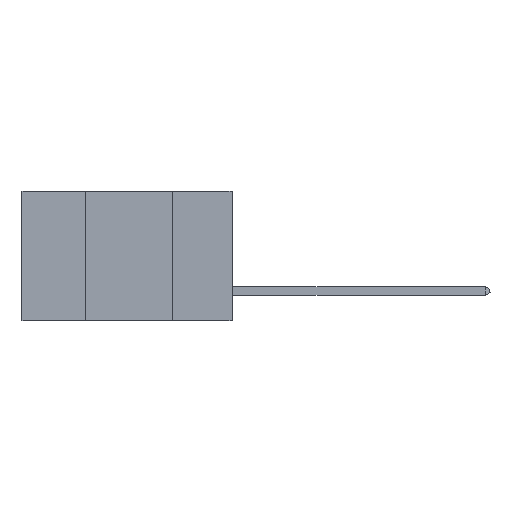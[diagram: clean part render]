
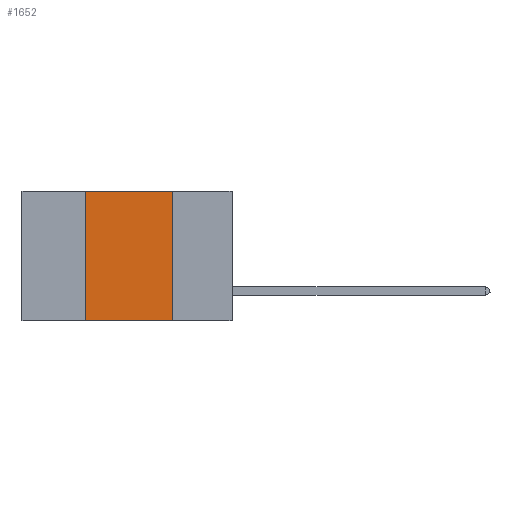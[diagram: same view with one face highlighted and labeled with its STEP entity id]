
A CAD part, left-side view. The second image highlights one B-rep face of the part: STEP entity #1652.
In plain terms, the highlighted planar face has unit normal (-1, 0, 0).
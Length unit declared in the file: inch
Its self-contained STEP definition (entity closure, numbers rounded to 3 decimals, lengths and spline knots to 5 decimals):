
#107 = PLANE ( 'NONE',  #6548 ) ;
#110 = VERTEX_POINT ( 'NONE', #2593 ) ;
#738 = ORIENTED_EDGE ( 'NONE', *, *, #14690, .T. ) ;
#1109 = LINE ( 'NONE', #14094, #13991 ) ;
#1227 = CARTESIAN_POINT ( 'NONE',  ( 0., 0.17, 0. ) ) ;
#1652 = ADVANCED_FACE ( 'NONE', ( #6645 ), #107, .F. ) ;
#2269 = ORIENTED_EDGE ( 'NONE', *, *, #9632, .F. ) ;
#2276 = VERTEX_POINT ( 'NONE', #3447 ) ;
#2307 = EDGE_CURVE ( 'NONE', #13519, #12713, #13987, .T. ) ;
#2593 = CARTESIAN_POINT ( 'NONE',  ( 0., 0.42, -0.37 ) ) ;
#3060 = LINE ( 'NONE', #14406, #4971 ) ;
#3086 = EDGE_CURVE ( 'NONE', #110, #2276, #1109, .T. ) ;
#3099 = EDGE_LOOP ( 'NONE', ( #4401, #2269, #9036, #738 ) ) ;
#3417 = DIRECTION ( 'NONE',  ( 0., -1., 0. ) ) ;
#3447 = CARTESIAN_POINT ( 'NONE',  ( 0., 0.42, 0. ) ) ;
#3971 = DIRECTION ( 'NONE',  ( 1., 0., 0. ) ) ;
#4401 = ORIENTED_EDGE ( 'NONE', *, *, #2307, .F. ) ;
#4971 = VECTOR ( 'NONE', #6022, 39.37008 ) ;
#5076 = CARTESIAN_POINT ( 'NONE',  ( 0., 0.6, 0. ) ) ;
#5434 = CARTESIAN_POINT ( 'NONE',  ( 0., 0.17, -0.37 ) ) ;
#5524 = DIRECTION ( 'NONE',  ( 0., 0., 1. ) ) ;
#6022 = DIRECTION ( 'NONE',  ( 0., -1., 0. ) ) ;
#6548 = AXIS2_PLACEMENT_3D ( 'NONE', #5076, #3971, #14720 ) ;
#6645 = FACE_OUTER_BOUND ( 'NONE', #3099, .T. ) ;
#8882 = DIRECTION ( 'NONE',  ( 0., 0., -1. ) ) ;
#9036 = ORIENTED_EDGE ( 'NONE', *, *, #3086, .F. ) ;
#9523 = LINE ( 'NONE', #10779, #13104 ) ;
#9632 = EDGE_CURVE ( 'NONE', #2276, #13519, #9523, .T. ) ;
#10779 = CARTESIAN_POINT ( 'NONE',  ( 0., 0.6, 0. ) ) ;
#11206 = CARTESIAN_POINT ( 'NONE',  ( 0., 0.17, 0. ) ) ;
#12713 = VERTEX_POINT ( 'NONE', #5434 ) ;
#13104 = VECTOR ( 'NONE', #3417, 39.37008 ) ;
#13519 = VERTEX_POINT ( 'NONE', #1227 ) ;
#13987 = LINE ( 'NONE', #11206, #15713 ) ;
#13991 = VECTOR ( 'NONE', #5524, 39.37008 ) ;
#14094 = CARTESIAN_POINT ( 'NONE',  ( 0., 0.42, 0. ) ) ;
#14406 = CARTESIAN_POINT ( 'NONE',  ( 0., 0.6, -0.37 ) ) ;
#14690 = EDGE_CURVE ( 'NONE', #110, #12713, #3060, .T. ) ;
#14720 = DIRECTION ( 'NONE',  ( 0., 0., -1. ) ) ;
#15713 = VECTOR ( 'NONE', #8882, 39.37008 ) ;
